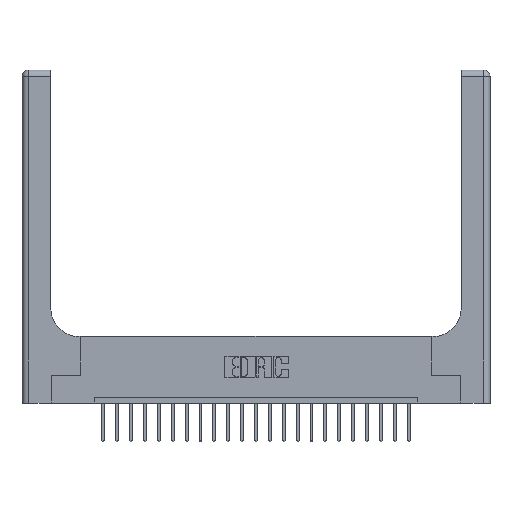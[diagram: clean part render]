
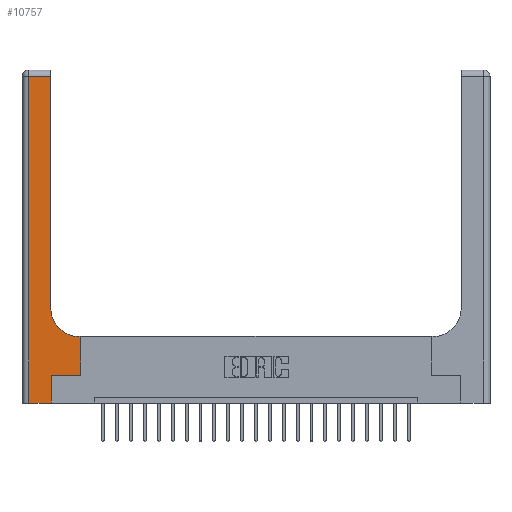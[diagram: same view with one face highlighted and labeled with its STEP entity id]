
A CAD part, top view. The second image highlights one B-rep face of the part: STEP entity #10757.
In plain terms, the highlighted planar face has unit normal (0, 0, 1).
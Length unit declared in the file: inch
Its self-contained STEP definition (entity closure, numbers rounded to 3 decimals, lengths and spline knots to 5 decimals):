
#261 = LINE ( 'NONE', #6284, #8781 ) ;
#476 = DIRECTION ( 'NONE',  ( 0., 1., 0. ) ) ;
#602 = LINE ( 'NONE', #10456, #5190 ) ;
#1151 = CIRCLE ( 'NONE', #1515, 0.25 ) ;
#1338 = VERTEX_POINT ( 'NONE', #21807 ) ;
#1515 = AXIS2_PLACEMENT_3D ( 'NONE', #2053, #17412, #7260 ) ;
#1713 = ORIENTED_EDGE ( 'NONE', *, *, #20953, .T. ) ;
#2053 = CARTESIAN_POINT ( 'NONE',  ( 0.51, 0.85, 0.37 ) ) ;
#2453 = ORIENTED_EDGE ( 'NONE', *, *, #11034, .T. ) ;
#2620 = CARTESIAN_POINT ( 'NONE',  ( 0.06, 3., 0.37 ) ) ;
#3726 = EDGE_CURVE ( 'NONE', #21958, #4085, #15596, .T. ) ;
#3794 = LINE ( 'NONE', #19146, #8068 ) ;
#4085 = VERTEX_POINT ( 'NONE', #12244 ) ;
#4682 = DIRECTION ( 'NONE',  ( 0., 0., -1. ) ) ;
#5190 = VECTOR ( 'NONE', #476, 39.37008 ) ;
#5242 = CARTESIAN_POINT ( 'NONE',  ( 0.06, 0., 0.37 ) ) ;
#5365 = EDGE_CURVE ( 'NONE', #12117, #5946, #1151, .T. ) ;
#5421 = CARTESIAN_POINT ( 'NONE',  ( 0.26, 0.6, 0.37 ) ) ;
#5623 = ORIENTED_EDGE ( 'NONE', *, *, #3726, .T. ) ;
#5930 = DIRECTION ( 'NONE',  ( 1., 0., 0. ) ) ;
#5946 = VERTEX_POINT ( 'NONE', #21089 ) ;
#5971 = DIRECTION ( 'NONE',  ( 0., -1., 0. ) ) ;
#5993 = ORIENTED_EDGE ( 'NONE', *, *, #15031, .T. ) ;
#6284 = CARTESIAN_POINT ( 'NONE',  ( 0.26, 3., 0.37 ) ) ;
#6585 = CARTESIAN_POINT ( 'NONE',  ( 0., 3., 0.37 ) ) ;
#6591 = VECTOR ( 'NONE', #11179, 39.37008 ) ;
#6669 = PLANE ( 'NONE',  #11571 ) ;
#7074 = ORIENTED_EDGE ( 'NONE', *, *, #10460, .T. ) ;
#7260 = DIRECTION ( 'NONE',  ( 1., 0., 0. ) ) ;
#8068 = VECTOR ( 'NONE', #9002, 39.37008 ) ;
#8214 = ORIENTED_EDGE ( 'NONE', *, *, #20881, .T. ) ;
#8343 = VECTOR ( 'NONE', #21942, 39.37008 ) ;
#8380 = ORIENTED_EDGE ( 'NONE', *, *, #5365, .T. ) ;
#8781 = VECTOR ( 'NONE', #13219, 39.37008 ) ;
#8888 = DIRECTION ( 'NONE',  ( -1., 0., 0. ) ) ;
#9002 = DIRECTION ( 'NONE',  ( 0., 1., 0. ) ) ;
#9039 = LINE ( 'NONE', #2620, #13056 ) ;
#10268 = ORIENTED_EDGE ( 'NONE', *, *, #18806, .T. ) ;
#10455 = VERTEX_POINT ( 'NONE', #11429 ) ;
#10456 = CARTESIAN_POINT ( 'NONE',  ( 0.265, 0., 0.37 ) ) ;
#10460 = EDGE_CURVE ( 'NONE', #5946, #11402, #261, .T. ) ;
#10667 = CARTESIAN_POINT ( 'NONE',  ( 0.51, 0.6, 0.37 ) ) ;
#10757 = ADVANCED_FACE ( 'NONE', ( #12248 ), #6669, .F. ) ;
#10841 = LINE ( 'NONE', #13131, #6591 ) ;
#11034 = EDGE_CURVE ( 'NONE', #1338, #21958, #9039, .T. ) ;
#11179 = DIRECTION ( 'NONE',  ( -1., 0., 0. ) ) ;
#11402 = VERTEX_POINT ( 'NONE', #18493 ) ;
#11429 = CARTESIAN_POINT ( 'NONE',  ( 0.528, 0.6, 0.37 ) ) ;
#11571 = AXIS2_PLACEMENT_3D ( 'NONE', #6585, #4682, #21746 ) ;
#12117 = VERTEX_POINT ( 'NONE', #10667 ) ;
#12244 = CARTESIAN_POINT ( 'NONE',  ( 0.265, 0., 0.37 ) ) ;
#12248 = FACE_OUTER_BOUND ( 'NONE', #20003, .T. ) ;
#12337 = CARTESIAN_POINT ( 'NONE',  ( 0.528, 0.25, 0.37 ) ) ;
#13056 = VECTOR ( 'NONE', #5971, 39.37008 ) ;
#13131 = CARTESIAN_POINT ( 'NONE',  ( 0., 2.94, 0.37 ) ) ;
#13219 = DIRECTION ( 'NONE',  ( 0., 1., 0. ) ) ;
#14028 = VECTOR ( 'NONE', #5930, 39.37008 ) ;
#14621 = CARTESIAN_POINT ( 'NONE',  ( 0., 0., 0.37 ) ) ;
#15031 = EDGE_CURVE ( 'NONE', #16821, #15714, #15768, .T. ) ;
#15254 = CARTESIAN_POINT ( 'NONE',  ( 0.265, 0.25, 0.37 ) ) ;
#15316 = EDGE_CURVE ( 'NONE', #15714, #10455, #3794, .T. ) ;
#15596 = LINE ( 'NONE', #14621, #14028 ) ;
#15714 = VERTEX_POINT ( 'NONE', #12337 ) ;
#15768 = LINE ( 'NONE', #15254, #8343 ) ;
#16821 = VERTEX_POINT ( 'NONE', #20900 ) ;
#17412 = DIRECTION ( 'NONE',  ( 0., 0., -1. ) ) ;
#18156 = VECTOR ( 'NONE', #8888, 39.37008 ) ;
#18493 = CARTESIAN_POINT ( 'NONE',  ( 0.26, 2.94, 0.37 ) ) ;
#18806 = EDGE_CURVE ( 'NONE', #11402, #1338, #10841, .T. ) ;
#19146 = CARTESIAN_POINT ( 'NONE',  ( 0.528, 0.25, 0.37 ) ) ;
#20003 = EDGE_LOOP ( 'NONE', ( #7074, #10268, #2453, #5623, #8214, #5993, #20006, #1713, #8380 ) ) ;
#20006 = ORIENTED_EDGE ( 'NONE', *, *, #15316, .T. ) ;
#20881 = EDGE_CURVE ( 'NONE', #4085, #16821, #602, .T. ) ;
#20900 = CARTESIAN_POINT ( 'NONE',  ( 0.265, 0.25, 0.37 ) ) ;
#20953 = EDGE_CURVE ( 'NONE', #10455, #12117, #21914, .T. ) ;
#21089 = CARTESIAN_POINT ( 'NONE',  ( 0.26, 0.85, 0.37 ) ) ;
#21746 = DIRECTION ( 'NONE',  ( -1., 0., 0. ) ) ;
#21807 = CARTESIAN_POINT ( 'NONE',  ( 0.06, 2.94, 0.37 ) ) ;
#21914 = LINE ( 'NONE', #5421, #18156 ) ;
#21942 = DIRECTION ( 'NONE',  ( 1., 0., 0. ) ) ;
#21958 = VERTEX_POINT ( 'NONE', #5242 ) ;
